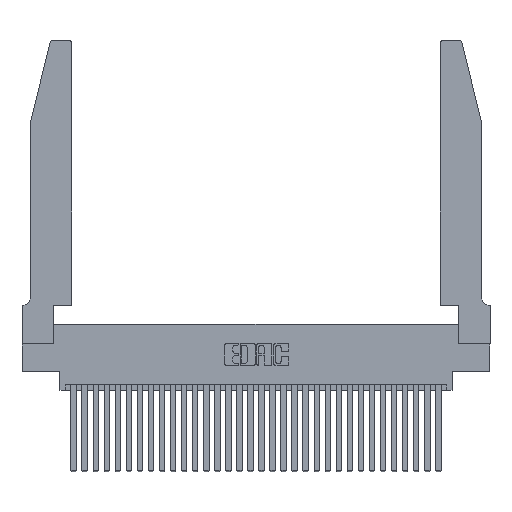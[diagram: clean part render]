
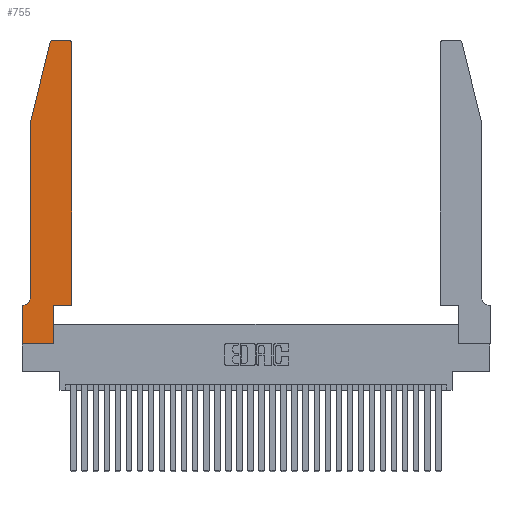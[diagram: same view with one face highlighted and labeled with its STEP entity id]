
A CAD part, top view. The second image highlights one B-rep face of the part: STEP entity #755.
In plain terms, the highlighted planar face has unit normal (0, 0, 1).
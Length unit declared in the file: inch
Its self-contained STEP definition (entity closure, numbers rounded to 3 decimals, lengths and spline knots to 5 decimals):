
#95 = ORIENTED_EDGE ( 'NONE', *, *, #14939, .T. ) ;
#705 = CARTESIAN_POINT ( 'NONE',  ( 0.4205, 2.75, 0.37 ) ) ;
#755 = ADVANCED_FACE ( 'NONE', ( #31537 ), #11017, .T. ) ;
#1812 = VERTEX_POINT ( 'NONE', #16024 ) ;
#1909 = CARTESIAN_POINT ( 'NONE',  ( 0.2605, 2.75, 0.37 ) ) ;
#1954 = CARTESIAN_POINT ( 'NONE',  ( 0.0755, 2., 0.37 ) ) ;
#2868 = CARTESIAN_POINT ( 'NONE',  ( 0.284, 2.72, 0.37 ) ) ;
#3104 = EDGE_CURVE ( 'NONE', #29845, #8866, #12992, .T. ) ;
#3621 = EDGE_CURVE ( 'NONE', #10916, #26588, #8597, .T. ) ;
#3984 = CARTESIAN_POINT ( 'NONE',  ( 0.2865, 0.35, 0.37 ) ) ;
#4537 = ORIENTED_EDGE ( 'NONE', *, *, #7746, .T. ) ;
#4605 = CARTESIAN_POINT ( 'NONE',  ( 0., 0.35, 0.37 ) ) ;
#5277 = VERTEX_POINT ( 'NONE', #705 ) ;
#5501 = DIRECTION ( 'NONE',  ( 0., 1., 0. ) ) ;
#5516 = DIRECTION ( 'NONE',  ( 0., 0., 1. ) ) ;
#5644 = DIRECTION ( 'NONE',  ( 0., 0., 1. ) ) ;
#5669 = DIRECTION ( 'NONE',  ( 1., 0., 0. ) ) ;
#6003 = LINE ( 'NONE', #25992, #24908 ) ;
#6177 = LINE ( 'NONE', #21100, #14049 ) ;
#6592 = VERTEX_POINT ( 'NONE', #15352 ) ;
#6753 = CARTESIAN_POINT ( 'NONE',  ( 0.0755, 2., 0.37 ) ) ;
#6969 = VERTEX_POINT ( 'NONE', #1954 ) ;
#7330 = DIRECTION ( 'NONE',  ( 0., 1., 0. ) ) ;
#7730 = LINE ( 'NONE', #8755, #27006 ) ;
#7746 = EDGE_CURVE ( 'NONE', #1812, #8612, #15536, .T. ) ;
#7957 = CARTESIAN_POINT ( 'NONE',  ( 0.2865, 0., 0.37 ) ) ;
#8236 = EDGE_CURVE ( 'NONE', #12304, #10916, #30385, .T. ) ;
#8484 = CARTESIAN_POINT ( 'NONE',  ( 0.2865, 0.35, 0.37 ) ) ;
#8597 = LINE ( 'NONE', #3984, #12964 ) ;
#8612 = VERTEX_POINT ( 'NONE', #22844 ) ;
#8649 = CIRCLE ( 'NONE', #26926, 0.07 ) ;
#8660 = EDGE_CURVE ( 'NONE', #26588, #29845, #6003, .T. ) ;
#8701 = VECTOR ( 'NONE', #9162, 39.37008 ) ;
#8755 = CARTESIAN_POINT ( 'NONE',  ( 0.0755, 2., 0.37 ) ) ;
#8866 = VERTEX_POINT ( 'NONE', #26872 ) ;
#9162 = DIRECTION ( 'NONE',  ( 0., -1., 0. ) ) ;
#9868 = VERTEX_POINT ( 'NONE', #25915 ) ;
#10916 = VERTEX_POINT ( 'NONE', #7957 ) ;
#11017 = PLANE ( 'NONE',  #25040 ) ;
#11343 = EDGE_CURVE ( 'NONE', #6592, #9868, #8649, .T. ) ;
#12082 = CARTESIAN_POINT ( 'NONE',  ( 0.4505, 0.35, 0.37 ) ) ;
#12304 = VERTEX_POINT ( 'NONE', #13273 ) ;
#12564 = ORIENTED_EDGE ( 'NONE', *, *, #31602, .T. ) ;
#12636 = ORIENTED_EDGE ( 'NONE', *, *, #27019, .T. ) ;
#12789 = ORIENTED_EDGE ( 'NONE', *, *, #11343, .T. ) ;
#12964 = VECTOR ( 'NONE', #5501, 39.37008 ) ;
#12992 = LINE ( 'NONE', #12082, #24777 ) ;
#13196 = ORIENTED_EDGE ( 'NONE', *, *, #20623, .T. ) ;
#13273 = CARTESIAN_POINT ( 'NONE',  ( 0., 0., 0.37 ) ) ;
#13416 = DIRECTION ( 'NONE',  ( -1., 0., 0. ) ) ;
#13527 = EDGE_CURVE ( 'NONE', #8612, #6969, #7730, .T. ) ;
#13572 = CARTESIAN_POINT ( 'NONE',  ( 0., 0.35, 0.37 ) ) ;
#13928 = LINE ( 'NONE', #1909, #25326 ) ;
#14049 = VECTOR ( 'NONE', #13416, 39.37008 ) ;
#14613 = CARTESIAN_POINT ( 'NONE',  ( 0., 0., 0.37 ) ) ;
#14939 = EDGE_CURVE ( 'NONE', #5277, #1812, #13928, .T. ) ;
#15352 = CARTESIAN_POINT ( 'NONE',  ( 0.0755, 0.42, 0.37 ) ) ;
#15536 = CIRCLE ( 'NONE', #24153, 0.03 ) ;
#15743 = VERTEX_POINT ( 'NONE', #4605 ) ;
#15872 = DIRECTION ( 'NONE',  ( 1., 0., 0. ) ) ;
#16024 = CARTESIAN_POINT ( 'NONE',  ( 0.284, 2.75, 0.37 ) ) ;
#16300 = EDGE_CURVE ( 'NONE', #6969, #6592, #22120, .T. ) ;
#17397 = DIRECTION ( 'NONE',  ( -1., 0., 0. ) ) ;
#18352 = CARTESIAN_POINT ( 'NONE',  ( 0., 0., 0.37 ) ) ;
#18452 = ORIENTED_EDGE ( 'NONE', *, *, #3621, .T. ) ;
#18899 = AXIS2_PLACEMENT_3D ( 'NONE', #24977, #5516, #23123 ) ;
#19423 = VECTOR ( 'NONE', #30831, 39.37008 ) ;
#19470 = ORIENTED_EDGE ( 'NONE', *, *, #8236, .T. ) ;
#19503 = ORIENTED_EDGE ( 'NONE', *, *, #8660, .T. ) ;
#20470 = DIRECTION ( 'NONE',  ( 0., 0., 1. ) ) ;
#20597 = ORIENTED_EDGE ( 'NONE', *, *, #3104, .T. ) ;
#20623 = EDGE_CURVE ( 'NONE', #15743, #12304, #26060, .T. ) ;
#20715 = EDGE_LOOP ( 'NONE', ( #95, #4537, #23412, #24603, #12789, #12564, #13196, #19470, #18452, #19503, #20597, #12636 ) ) ;
#21100 = CARTESIAN_POINT ( 'NONE',  ( 0.0755, 0.35, 0.37 ) ) ;
#21863 = CIRCLE ( 'NONE', #18899, 0.03 ) ;
#22120 = LINE ( 'NONE', #6753, #8701 ) ;
#22844 = CARTESIAN_POINT ( 'NONE',  ( 0.25487, 2.72718, 0.37 ) ) ;
#23123 = DIRECTION ( 'NONE',  ( 1., 0., 0. ) ) ;
#23412 = ORIENTED_EDGE ( 'NONE', *, *, #13527, .T. ) ;
#23743 = VECTOR ( 'NONE', #26701, 39.37008 ) ;
#24153 = AXIS2_PLACEMENT_3D ( 'NONE', #2868, #20470, #30299 ) ;
#24603 = ORIENTED_EDGE ( 'NONE', *, *, #16300, .T. ) ;
#24777 = VECTOR ( 'NONE', #7330, 39.37008 ) ;
#24908 = VECTOR ( 'NONE', #5669, 39.37008 ) ;
#24977 = CARTESIAN_POINT ( 'NONE',  ( 0.4205, 2.72, 0.37 ) ) ;
#25040 = AXIS2_PLACEMENT_3D ( 'NONE', #13572, #5644, #15872 ) ;
#25326 = VECTOR ( 'NONE', #29445, 39.37008 ) ;
#25915 = CARTESIAN_POINT ( 'NONE',  ( 0.0055, 0.35, 0.37 ) ) ;
#25992 = CARTESIAN_POINT ( 'NONE',  ( 0.4505, 0.35, 0.37 ) ) ;
#26060 = LINE ( 'NONE', #18352, #19423 ) ;
#26588 = VERTEX_POINT ( 'NONE', #8484 ) ;
#26701 = DIRECTION ( 'NONE',  ( 1., 0., 0. ) ) ;
#26872 = CARTESIAN_POINT ( 'NONE',  ( 0.4505, 2.72, 0.37 ) ) ;
#26926 = AXIS2_PLACEMENT_3D ( 'NONE', #29658, #32294, #17397 ) ;
#27006 = VECTOR ( 'NONE', #31253, 39.37008 ) ;
#27019 = EDGE_CURVE ( 'NONE', #8866, #5277, #21863, .T. ) ;
#28858 = CARTESIAN_POINT ( 'NONE',  ( 0.4505, 0.35, 0.37 ) ) ;
#29445 = DIRECTION ( 'NONE',  ( -1., 0., 0. ) ) ;
#29658 = CARTESIAN_POINT ( 'NONE',  ( 0.0055, 0.42, 0.37 ) ) ;
#29845 = VERTEX_POINT ( 'NONE', #28858 ) ;
#30299 = DIRECTION ( 'NONE',  ( 1., 0., 0. ) ) ;
#30385 = LINE ( 'NONE', #14613, #23743 ) ;
#30831 = DIRECTION ( 'NONE',  ( 0., -1., 0. ) ) ;
#31253 = DIRECTION ( 'NONE',  ( -0.239, -0.971, 0. ) ) ;
#31537 = FACE_OUTER_BOUND ( 'NONE', #20715, .T. ) ;
#31602 = EDGE_CURVE ( 'NONE', #9868, #15743, #6177, .T. ) ;
#32294 = DIRECTION ( 'NONE',  ( 0., 0., -1. ) ) ;
